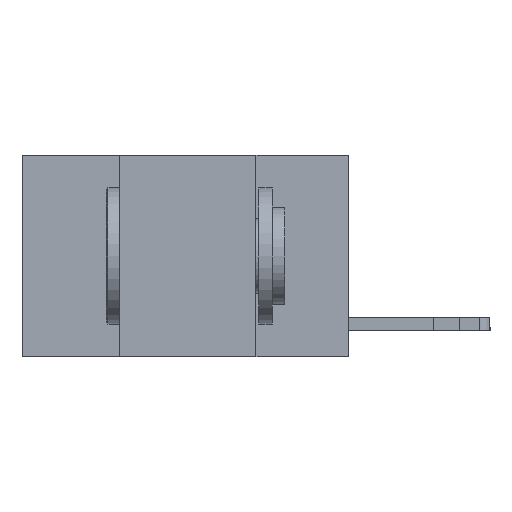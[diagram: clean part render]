
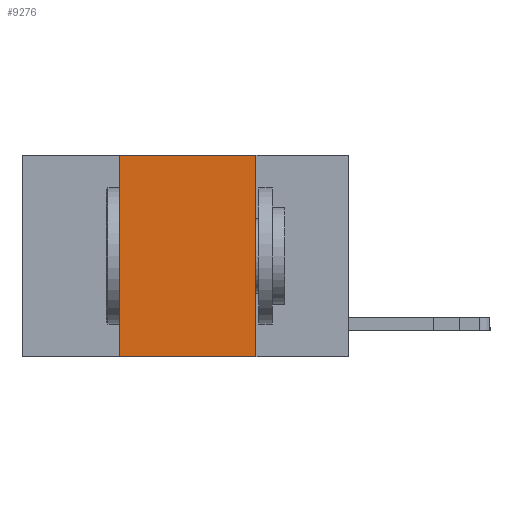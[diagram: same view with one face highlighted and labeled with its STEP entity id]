
A CAD part, left-side view. The second image highlights one B-rep face of the part: STEP entity #9276.
In plain terms, the highlighted planar face has unit normal (-1, 0, 0).
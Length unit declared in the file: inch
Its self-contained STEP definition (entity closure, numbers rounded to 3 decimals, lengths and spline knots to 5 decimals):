
#915 = CARTESIAN_POINT ( 'NONE',  ( 0., 0.6, 0. ) ) ;
#1495 = CARTESIAN_POINT ( 'NONE',  ( 0., 0.42, 0. ) ) ;
#1933 = VERTEX_POINT ( 'NONE', #21797 ) ;
#2437 = LINE ( 'NONE', #2548, #4817 ) ;
#2548 = CARTESIAN_POINT ( 'NONE',  ( 0., 0.6, -0.37 ) ) ;
#3547 = LINE ( 'NONE', #1495, #9580 ) ;
#3912 = VECTOR ( 'NONE', #16466, 39.37008 ) ;
#4117 = VERTEX_POINT ( 'NONE', #19336 ) ;
#4562 = EDGE_LOOP ( 'NONE', ( #12510, #14708, #8934, #17626 ) ) ;
#4593 = VECTOR ( 'NONE', #18059, 39.37008 ) ;
#4817 = VECTOR ( 'NONE', #21606, 39.37008 ) ;
#5354 = DIRECTION ( 'NONE',  ( 0., 0., 1. ) ) ;
#5483 = EDGE_CURVE ( 'NONE', #18384, #4117, #2437, .T. ) ;
#7775 = AXIS2_PLACEMENT_3D ( 'NONE', #10442, #10544, #13948 ) ;
#8934 = ORIENTED_EDGE ( 'NONE', *, *, #21216, .F. ) ;
#9276 = ADVANCED_FACE ( 'NONE', ( #16917 ), #13386, .F. ) ;
#9326 = CARTESIAN_POINT ( 'NONE',  ( 0., 0.17, 0. ) ) ;
#9580 = VECTOR ( 'NONE', #5354, 39.37008 ) ;
#9780 = CARTESIAN_POINT ( 'NONE',  ( 0., 0.42, -0.37 ) ) ;
#10442 = CARTESIAN_POINT ( 'NONE',  ( 0., 0.6, 0. ) ) ;
#10544 = DIRECTION ( 'NONE',  ( 1., 0., 0. ) ) ;
#11721 = EDGE_CURVE ( 'NONE', #1933, #16403, #17605, .T. ) ;
#12510 = ORIENTED_EDGE ( 'NONE', *, *, #14828, .F. ) ;
#13386 = PLANE ( 'NONE',  #7775 ) ;
#13948 = DIRECTION ( 'NONE',  ( 0., 0., -1. ) ) ;
#14708 = ORIENTED_EDGE ( 'NONE', *, *, #11721, .F. ) ;
#14828 = EDGE_CURVE ( 'NONE', #16403, #4117, #21469, .T. ) ;
#16403 = VERTEX_POINT ( 'NONE', #21168 ) ;
#16466 = DIRECTION ( 'NONE',  ( 0., 0., -1. ) ) ;
#16917 = FACE_OUTER_BOUND ( 'NONE', #4562, .T. ) ;
#17605 = LINE ( 'NONE', #915, #4593 ) ;
#17626 = ORIENTED_EDGE ( 'NONE', *, *, #5483, .T. ) ;
#18059 = DIRECTION ( 'NONE',  ( 0., -1., 0. ) ) ;
#18384 = VERTEX_POINT ( 'NONE', #9780 ) ;
#19336 = CARTESIAN_POINT ( 'NONE',  ( 0., 0.17, -0.37 ) ) ;
#21168 = CARTESIAN_POINT ( 'NONE',  ( 0., 0.17, 0. ) ) ;
#21216 = EDGE_CURVE ( 'NONE', #18384, #1933, #3547, .T. ) ;
#21469 = LINE ( 'NONE', #9326, #3912 ) ;
#21606 = DIRECTION ( 'NONE',  ( 0., -1., 0. ) ) ;
#21797 = CARTESIAN_POINT ( 'NONE',  ( 0., 0.42, 0. ) ) ;
